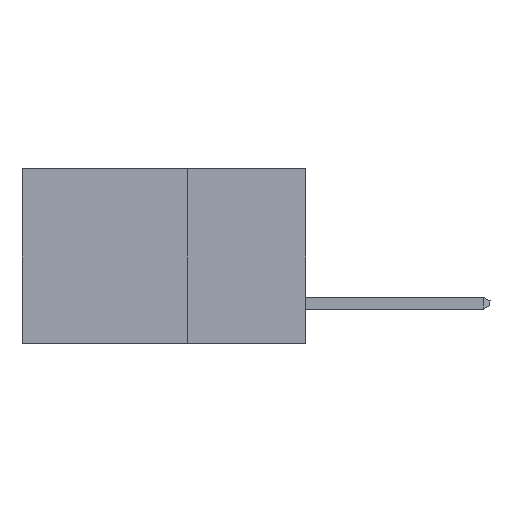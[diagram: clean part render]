
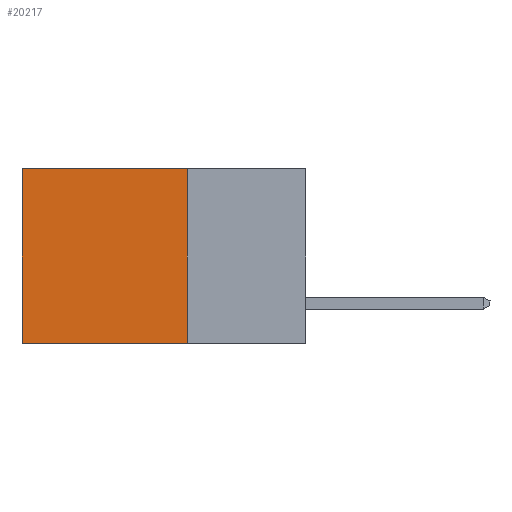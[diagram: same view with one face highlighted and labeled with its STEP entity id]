
A CAD part, left-side view. The second image highlights one B-rep face of the part: STEP entity #20217.
In plain terms, the highlighted planar face has unit normal (-1, 0, 0).
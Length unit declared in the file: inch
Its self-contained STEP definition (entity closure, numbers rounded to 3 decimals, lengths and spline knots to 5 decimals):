
#546 = CARTESIAN_POINT ( 'NONE',  ( 0.2615, 0.6, -0.37 ) ) ;
#1738 = PLANE ( 'NONE',  #11203 ) ;
#3819 = DIRECTION ( 'NONE',  ( 0., 1., 0. ) ) ;
#4128 = EDGE_CURVE ( 'NONE', #16245, #4449, #14842, .T. ) ;
#4449 = VERTEX_POINT ( 'NONE', #16569 ) ;
#5182 = EDGE_LOOP ( 'NONE', ( #6197, #6556, #6448, #18702 ) ) ;
#6197 = ORIENTED_EDGE ( 'NONE', *, *, #16459, .T. ) ;
#6448 = ORIENTED_EDGE ( 'NONE', *, *, #10927, .F. ) ;
#6556 = ORIENTED_EDGE ( 'NONE', *, *, #4128, .F. ) ;
#6756 = LINE ( 'NONE', #19701, #18581 ) ;
#6790 = LINE ( 'NONE', #10415, #13453 ) ;
#7333 = LINE ( 'NONE', #546, #12143 ) ;
#7664 = VECTOR ( 'NONE', #10239, 39.37008 ) ;
#8076 = CARTESIAN_POINT ( 'NONE',  ( 0.2615, 0.6, 0. ) ) ;
#8122 = DIRECTION ( 'NONE',  ( 1., 0., 0. ) ) ;
#9442 = CARTESIAN_POINT ( 'NONE',  ( 0.2615, 0.25, -0.37 ) ) ;
#10239 = DIRECTION ( 'NONE',  ( 0., 1., 0. ) ) ;
#10415 = CARTESIAN_POINT ( 'NONE',  ( 0.2615, 0.25, -0.37 ) ) ;
#10927 = EDGE_CURVE ( 'NONE', #14185, #16245, #6790, .T. ) ;
#11054 = FACE_OUTER_BOUND ( 'NONE', #5182, .T. ) ;
#11203 = AXIS2_PLACEMENT_3D ( 'NONE', #15873, #8122, #14490 ) ;
#12143 = VECTOR ( 'NONE', #18292, 39.37008 ) ;
#12190 = DIRECTION ( 'NONE',  ( 0., 0., -1. ) ) ;
#13453 = VECTOR ( 'NONE', #12190, 39.37008 ) ;
#14185 = VERTEX_POINT ( 'NONE', #16797 ) ;
#14490 = DIRECTION ( 'NONE',  ( 0., 0., -1. ) ) ;
#14842 = LINE ( 'NONE', #17974, #7664 ) ;
#15873 = CARTESIAN_POINT ( 'NONE',  ( 0.2615, 0.25, -0.37 ) ) ;
#16245 = VERTEX_POINT ( 'NONE', #9442 ) ;
#16459 = EDGE_CURVE ( 'NONE', #19778, #4449, #7333, .T. ) ;
#16569 = CARTESIAN_POINT ( 'NONE',  ( 0.2615, 0.6, -0.37 ) ) ;
#16797 = CARTESIAN_POINT ( 'NONE',  ( 0.2615, 0.25, 0. ) ) ;
#17974 = CARTESIAN_POINT ( 'NONE',  ( 0.2615, 0.25, -0.37 ) ) ;
#18292 = DIRECTION ( 'NONE',  ( 0., 0., -1. ) ) ;
#18581 = VECTOR ( 'NONE', #3819, 39.37008 ) ;
#18702 = ORIENTED_EDGE ( 'NONE', *, *, #20265, .T. ) ;
#19701 = CARTESIAN_POINT ( 'NONE',  ( 0.2615, 0.25, 0. ) ) ;
#19778 = VERTEX_POINT ( 'NONE', #8076 ) ;
#20217 = ADVANCED_FACE ( 'NONE', ( #11054 ), #1738, .F. ) ;
#20265 = EDGE_CURVE ( 'NONE', #14185, #19778, #6756, .T. ) ;
